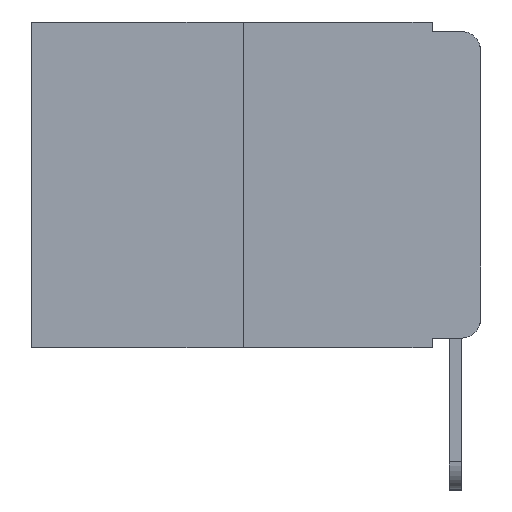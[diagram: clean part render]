
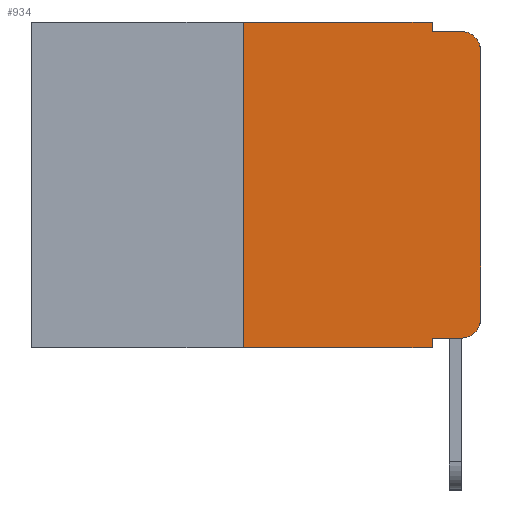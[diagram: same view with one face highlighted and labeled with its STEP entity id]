
A CAD part, left-side view. The second image highlights one B-rep face of the part: STEP entity #934.
In plain terms, the highlighted planar face has unit normal (-1, 0, 0).
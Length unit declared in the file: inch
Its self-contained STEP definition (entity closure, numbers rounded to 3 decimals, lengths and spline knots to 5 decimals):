
#451 = VECTOR ( 'NONE', #11717, 39.37008 ) ;
#934 = ADVANCED_FACE ( 'NONE', ( #10778 ), #8071, .F. ) ;
#1070 = LINE ( 'NONE', #11592, #5190 ) ;
#1281 = CARTESIAN_POINT ( 'NONE',  ( 0., 0.25, 0. ) ) ;
#1398 = LINE ( 'NONE', #6770, #14243 ) ;
#1496 = DIRECTION ( 'NONE',  ( 0., 0., -1. ) ) ;
#1729 = ORIENTED_EDGE ( 'NONE', *, *, #3671, .T. ) ;
#1901 = EDGE_CURVE ( 'NONE', #8740, #4631, #7509, .T. ) ;
#1906 = DIRECTION ( 'NONE',  ( 0., -1., 0. ) ) ;
#1927 = AXIS2_PLACEMENT_3D ( 'NONE', #11759, #2113, #13308 ) ;
#2073 = CARTESIAN_POINT ( 'NONE',  ( 0., 0.051, 0. ) ) ;
#2113 = DIRECTION ( 'NONE',  ( -1., 0., 0. ) ) ;
#2139 = DIRECTION ( 'NONE',  ( 0., -1., 0. ) ) ;
#2408 = VERTEX_POINT ( 'NONE', #8698 ) ;
#2882 = ORIENTED_EDGE ( 'NONE', *, *, #4037, .T. ) ;
#3160 = ORIENTED_EDGE ( 'NONE', *, *, #4132, .T. ) ;
#3434 = CARTESIAN_POINT ( 'NONE',  ( 0., 0.02, -0.01 ) ) ;
#3671 = EDGE_CURVE ( 'NONE', #18741, #12894, #1398, .T. ) ;
#3743 = CARTESIAN_POINT ( 'NONE',  ( 0., 0.051, 0. ) ) ;
#4037 = EDGE_CURVE ( 'NONE', #4040, #2408, #18905, .T. ) ;
#4040 = VERTEX_POINT ( 'NONE', #16023 ) ;
#4063 = EDGE_CURVE ( 'NONE', #7025, #4040, #1070, .T. ) ;
#4066 = EDGE_CURVE ( 'NONE', #7025, #12894, #17482, .T. ) ;
#4096 = EDGE_CURVE ( 'NONE', #18741, #8740, #12501, .T. ) ;
#4102 = EDGE_CURVE ( 'NONE', #4631, #7761, #16034, .T. ) ;
#4108 = EDGE_CURVE ( 'NONE', #7761, #19477, #19567, .T. ) ;
#4132 = EDGE_CURVE ( 'NONE', #12179, #19477, #12011, .T. ) ;
#4165 = EDGE_CURVE ( 'NONE', #2408, #12179, #18672, .T. ) ;
#4212 = VECTOR ( 'NONE', #5441, 39.37008 ) ;
#4631 = VERTEX_POINT ( 'NONE', #9660 ) ;
#5190 = VECTOR ( 'NONE', #1906, 39.37008 ) ;
#5373 = DIRECTION ( 'NONE',  ( 0., 0., -1. ) ) ;
#5428 = CARTESIAN_POINT ( 'NONE',  ( 0., 0.051, -0.333 ) ) ;
#5441 = DIRECTION ( 'NONE',  ( 0., 0., 1. ) ) ;
#6723 = ORIENTED_EDGE ( 'NONE', *, *, #4063, .T. ) ;
#6770 = CARTESIAN_POINT ( 'NONE',  ( 0., 0.473, -0.343 ) ) ;
#7025 = VERTEX_POINT ( 'NONE', #5428 ) ;
#7189 = DIRECTION ( 'NONE',  ( 0., 0., 1. ) ) ;
#7509 = LINE ( 'NONE', #7803, #15712 ) ;
#7761 = VERTEX_POINT ( 'NONE', #9405 ) ;
#7803 = CARTESIAN_POINT ( 'NONE',  ( 0., 0.473, 0. ) ) ;
#8071 = PLANE ( 'NONE',  #17586 ) ;
#8345 = DIRECTION ( 'NONE',  ( -1., 0., 0. ) ) ;
#8392 = CARTESIAN_POINT ( 'NONE',  ( 0., 0.051, -0.343 ) ) ;
#8698 = CARTESIAN_POINT ( 'NONE',  ( 0., 0., -0.313 ) ) ;
#8740 = VERTEX_POINT ( 'NONE', #1281 ) ;
#9405 = CARTESIAN_POINT ( 'NONE',  ( 0., 0.051, -0.01 ) ) ;
#9629 = CARTESIAN_POINT ( 'NONE',  ( 0., 0.473, 0. ) ) ;
#9660 = CARTESIAN_POINT ( 'NONE',  ( 0., 0.051, 0. ) ) ;
#10366 = ORIENTED_EDGE ( 'NONE', *, *, #4066, .F. ) ;
#10778 = FACE_OUTER_BOUND ( 'NONE', #14390, .T. ) ;
#10998 = AXIS2_PLACEMENT_3D ( 'NONE', #17581, #8345, #19065 ) ;
#11222 = DIRECTION ( 'NONE',  ( 1., 0., 0. ) ) ;
#11532 = VECTOR ( 'NONE', #2139, 39.37008 ) ;
#11592 = CARTESIAN_POINT ( 'NONE',  ( 0., 0.051, -0.333 ) ) ;
#11717 = DIRECTION ( 'NONE',  ( 0., 0., -1. ) ) ;
#11759 = CARTESIAN_POINT ( 'NONE',  ( 0., 0.02, -0.03 ) ) ;
#11892 = CARTESIAN_POINT ( 'NONE',  ( 0., 0.25, -0.343 ) ) ;
#12011 = CIRCLE ( 'NONE', #1927, 0.02 ) ;
#12179 = VERTEX_POINT ( 'NONE', #17690 ) ;
#12451 = DIRECTION ( 'NONE',  ( 0., -1., 0. ) ) ;
#12501 = LINE ( 'NONE', #16207, #4212 ) ;
#12894 = VERTEX_POINT ( 'NONE', #8392 ) ;
#13308 = DIRECTION ( 'NONE',  ( 0., 0., -1. ) ) ;
#14243 = VECTOR ( 'NONE', #15977, 39.37008 ) ;
#14390 = EDGE_LOOP ( 'NONE', ( #19180, #3160, #16101, #20098, #17080, #17554, #1729, #10366, #6723, #2882 ) ) ;
#14801 = CARTESIAN_POINT ( 'NONE',  ( 0., 0.051, -0.01 ) ) ;
#15712 = VECTOR ( 'NONE', #12451, 39.37008 ) ;
#15977 = DIRECTION ( 'NONE',  ( 0., -1., 0. ) ) ;
#16023 = CARTESIAN_POINT ( 'NONE',  ( 0., 0.02, -0.333 ) ) ;
#16034 = LINE ( 'NONE', #2073, #451 ) ;
#16101 = ORIENTED_EDGE ( 'NONE', *, *, #4108, .F. ) ;
#16207 = CARTESIAN_POINT ( 'NONE',  ( 0., 0.25, 0. ) ) ;
#17008 = VECTOR ( 'NONE', #5373, 39.37008 ) ;
#17080 = ORIENTED_EDGE ( 'NONE', *, *, #1901, .F. ) ;
#17482 = LINE ( 'NONE', #3743, #17008 ) ;
#17554 = ORIENTED_EDGE ( 'NONE', *, *, #4096, .F. ) ;
#17581 = CARTESIAN_POINT ( 'NONE',  ( 0., 0.02, -0.313 ) ) ;
#17586 = AXIS2_PLACEMENT_3D ( 'NONE', #9629, #11222, #1496 ) ;
#17690 = CARTESIAN_POINT ( 'NONE',  ( 0., 0., -0.03 ) ) ;
#17938 = CARTESIAN_POINT ( 'NONE',  ( 0., 0., 0. ) ) ;
#18207 = VECTOR ( 'NONE', #7189, 39.37008 ) ;
#18672 = LINE ( 'NONE', #17938, #18207 ) ;
#18741 = VERTEX_POINT ( 'NONE', #11892 ) ;
#18905 = CIRCLE ( 'NONE', #10998, 0.02 ) ;
#19065 = DIRECTION ( 'NONE',  ( 0., 0., -1. ) ) ;
#19180 = ORIENTED_EDGE ( 'NONE', *, *, #4165, .T. ) ;
#19477 = VERTEX_POINT ( 'NONE', #3434 ) ;
#19567 = LINE ( 'NONE', #14801, #11532 ) ;
#20098 = ORIENTED_EDGE ( 'NONE', *, *, #4102, .F. ) ;
